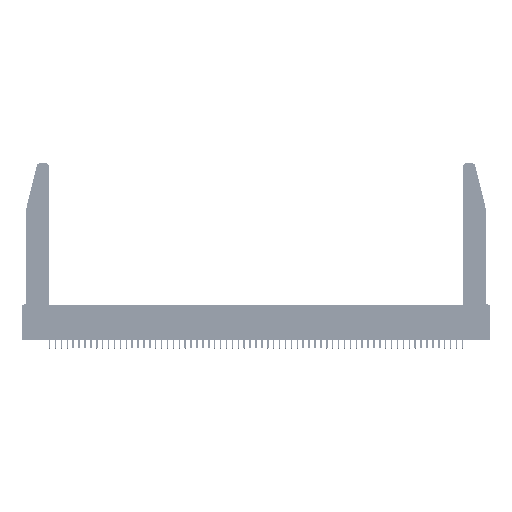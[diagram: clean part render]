
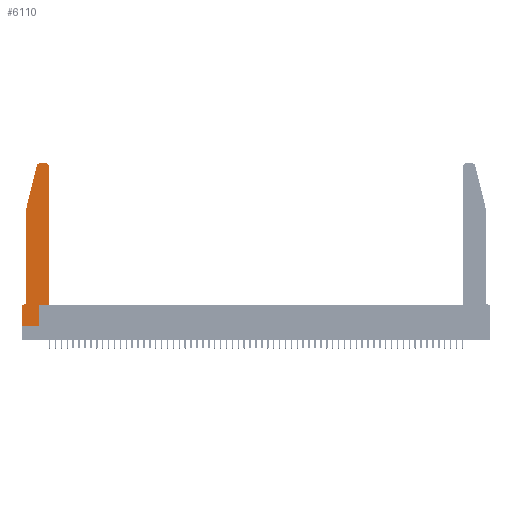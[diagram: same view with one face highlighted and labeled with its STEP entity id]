
A CAD part, top view. The second image highlights one B-rep face of the part: STEP entity #6110.
In plain terms, the highlighted planar face has unit normal (0, 0, 1).
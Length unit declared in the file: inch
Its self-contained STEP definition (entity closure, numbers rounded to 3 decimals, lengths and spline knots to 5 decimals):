
#269 = CARTESIAN_POINT ( 'NONE',  ( 0.0055, 0.42, 0.37 ) ) ;
#1552 = CARTESIAN_POINT ( 'NONE',  ( 0., 0., 0.37 ) ) ;
#1593 = DIRECTION ( 'NONE',  ( 1., 0., 0. ) ) ;
#1777 = ORIENTED_EDGE ( 'NONE', *, *, #32491, .T. ) ;
#1804 = CARTESIAN_POINT ( 'NONE',  ( 0.2865, 0.35, 0.37 ) ) ;
#2118 = VERTEX_POINT ( 'NONE', #39804 ) ;
#2926 = EDGE_CURVE ( 'NONE', #52305, #33235, #49611, .T. ) ;
#4724 = DIRECTION ( 'NONE',  ( -1., 0., 0. ) ) ;
#5284 = CARTESIAN_POINT ( 'NONE',  ( 0.4505, 2.72, 0.37 ) ) ;
#5709 = EDGE_CURVE ( 'NONE', #37300, #2118, #21955, .T. ) ;
#5731 = DIRECTION ( 'NONE',  ( -0.239, -0.971, 0. ) ) ;
#6020 = CARTESIAN_POINT ( 'NONE',  ( 0.284, 2.72, 0.37 ) ) ;
#6110 = ADVANCED_FACE ( 'NONE', ( #21896 ), #30469, .T. ) ;
#6280 = ORIENTED_EDGE ( 'NONE', *, *, #5709, .T. ) ;
#7182 = ORIENTED_EDGE ( 'NONE', *, *, #50861, .T. ) ;
#8205 = CARTESIAN_POINT ( 'NONE',  ( 0.4505, 0.35, 0.37 ) ) ;
#8643 = DIRECTION ( 'NONE',  ( 0., 0., 1. ) ) ;
#8698 = VECTOR ( 'NONE', #23076, 39.37008 ) ;
#10059 = LINE ( 'NONE', #27499, #8698 ) ;
#10401 = DIRECTION ( 'NONE',  ( 1., 0., 0. ) ) ;
#11007 = ORIENTED_EDGE ( 'NONE', *, *, #17487, .T. ) ;
#11427 = CARTESIAN_POINT ( 'NONE',  ( 0.25487, 2.72718, 0.37 ) ) ;
#12395 = LINE ( 'NONE', #8205, #22644 ) ;
#12562 = DIRECTION ( 'NONE',  ( 0., 1., 0. ) ) ;
#13392 = VECTOR ( 'NONE', #5731, 39.37008 ) ;
#13695 = CARTESIAN_POINT ( 'NONE',  ( 0.2865, 0.35, 0.37 ) ) ;
#14216 = ORIENTED_EDGE ( 'NONE', *, *, #37200, .T. ) ;
#14345 = LINE ( 'NONE', #44198, #24611 ) ;
#14688 = EDGE_LOOP ( 'NONE', ( #11007, #30832, #22617, #28702, #14216, #19615, #7182, #6280, #21599, #38607, #56515, #1777 ) ) ;
#16716 = DIRECTION ( 'NONE',  ( 1., 0., 0. ) ) ;
#17437 = VERTEX_POINT ( 'NONE', #35310 ) ;
#17487 = EDGE_CURVE ( 'NONE', #32050, #53850, #14345, .T. ) ;
#17672 = AXIS2_PLACEMENT_3D ( 'NONE', #53911, #27817, #1593 ) ;
#18965 = DIRECTION ( 'NONE',  ( 1., 0., 0. ) ) ;
#19210 = CIRCLE ( 'NONE', #37378, 0.07 ) ;
#19615 = ORIENTED_EDGE ( 'NONE', *, *, #27882, .T. ) ;
#20048 = CARTESIAN_POINT ( 'NONE',  ( 0., 0., 0.37 ) ) ;
#20575 = CARTESIAN_POINT ( 'NONE',  ( 0.0755, 0.35, 0.37 ) ) ;
#21590 = AXIS2_PLACEMENT_3D ( 'NONE', #6020, #36625, #10401 ) ;
#21599 = ORIENTED_EDGE ( 'NONE', *, *, #23009, .T. ) ;
#21896 = FACE_OUTER_BOUND ( 'NONE', #14688, .T. ) ;
#21955 = LINE ( 'NONE', #1552, #32270 ) ;
#22404 = DIRECTION ( 'NONE',  ( -1., 0., 0. ) ) ;
#22617 = ORIENTED_EDGE ( 'NONE', *, *, #2926, .T. ) ;
#22644 = VECTOR ( 'NONE', #12562, 39.37008 ) ;
#23009 = EDGE_CURVE ( 'NONE', #2118, #51243, #48115, .T. ) ;
#23076 = DIRECTION ( 'NONE',  ( 0., -1., 0. ) ) ;
#23194 = VECTOR ( 'NONE', #24442, 39.37008 ) ;
#24442 = DIRECTION ( 'NONE',  ( 0., -1., 0. ) ) ;
#24611 = VECTOR ( 'NONE', #22404, 39.37008 ) ;
#24880 = CIRCLE ( 'NONE', #17672, 0.03 ) ;
#25055 = LINE ( 'NONE', #38556, #35394 ) ;
#26169 = CIRCLE ( 'NONE', #21590, 0.03 ) ;
#27122 = CARTESIAN_POINT ( 'NONE',  ( 0.4505, 0.35, 0.37 ) ) ;
#27401 = LINE ( 'NONE', #20575, #39040 ) ;
#27499 = CARTESIAN_POINT ( 'NONE',  ( 0.0755, 2., 0.37 ) ) ;
#27817 = DIRECTION ( 'NONE',  ( 0., 0., 1. ) ) ;
#27882 = EDGE_CURVE ( 'NONE', #50797, #43122, #27401, .T. ) ;
#28244 = VERTEX_POINT ( 'NONE', #5284 ) ;
#28702 = ORIENTED_EDGE ( 'NONE', *, *, #33730, .T. ) ;
#30469 = PLANE ( 'NONE',  #50492 ) ;
#30832 = ORIENTED_EDGE ( 'NONE', *, *, #48964, .T. ) ;
#30971 = DIRECTION ( 'NONE',  ( 0., 0., -1. ) ) ;
#31197 = CARTESIAN_POINT ( 'NONE',  ( 0.284, 2.75, 0.37 ) ) ;
#32050 = VERTEX_POINT ( 'NONE', #38021 ) ;
#32270 = VECTOR ( 'NONE', #18965, 39.37008 ) ;
#32491 = EDGE_CURVE ( 'NONE', #28244, #32050, #24880, .T. ) ;
#33235 = VERTEX_POINT ( 'NONE', #41688 ) ;
#33644 = VERTEX_POINT ( 'NONE', #27122 ) ;
#33730 = EDGE_CURVE ( 'NONE', #33235, #17437, #10059, .T. ) ;
#34872 = CARTESIAN_POINT ( 'NONE',  ( 0., 0.35, 0.37 ) ) ;
#35310 = CARTESIAN_POINT ( 'NONE',  ( 0.0755, 0.42, 0.37 ) ) ;
#35394 = VECTOR ( 'NONE', #16716, 39.37008 ) ;
#36329 = CARTESIAN_POINT ( 'NONE',  ( 0.0755, 2., 0.37 ) ) ;
#36553 = VECTOR ( 'NONE', #41215, 39.37008 ) ;
#36625 = DIRECTION ( 'NONE',  ( 0., 0., 1. ) ) ;
#37200 = EDGE_CURVE ( 'NONE', #17437, #50797, #19210, .T. ) ;
#37300 = VERTEX_POINT ( 'NONE', #40097 ) ;
#37378 = AXIS2_PLACEMENT_3D ( 'NONE', #269, #30971, #4724 ) ;
#38021 = CARTESIAN_POINT ( 'NONE',  ( 0.4205, 2.75, 0.37 ) ) ;
#38172 = CARTESIAN_POINT ( 'NONE',  ( 0., 0.35, 0.37 ) ) ;
#38556 = CARTESIAN_POINT ( 'NONE',  ( 0.4505, 0.35, 0.37 ) ) ;
#38607 = ORIENTED_EDGE ( 'NONE', *, *, #46772, .T. ) ;
#39040 = VECTOR ( 'NONE', #51116, 39.37008 ) ;
#39230 = DIRECTION ( 'NONE',  ( 1., 0., 0. ) ) ;
#39804 = CARTESIAN_POINT ( 'NONE',  ( 0.2865, 0., 0.37 ) ) ;
#40097 = CARTESIAN_POINT ( 'NONE',  ( 0., 0., 0.37 ) ) ;
#41215 = DIRECTION ( 'NONE',  ( 0., 1., 0. ) ) ;
#41688 = CARTESIAN_POINT ( 'NONE',  ( 0.0755, 2., 0.37 ) ) ;
#43122 = VERTEX_POINT ( 'NONE', #38172 ) ;
#44198 = CARTESIAN_POINT ( 'NONE',  ( 0.2605, 2.75, 0.37 ) ) ;
#45011 = EDGE_CURVE ( 'NONE', #33644, #28244, #12395, .T. ) ;
#45603 = LINE ( 'NONE', #20048, #23194 ) ;
#46772 = EDGE_CURVE ( 'NONE', #51243, #33644, #25055, .T. ) ;
#48115 = LINE ( 'NONE', #1804, #36553 ) ;
#48964 = EDGE_CURVE ( 'NONE', #53850, #52305, #26169, .T. ) ;
#49436 = CARTESIAN_POINT ( 'NONE',  ( 0.0055, 0.35, 0.37 ) ) ;
#49611 = LINE ( 'NONE', #36329, #13392 ) ;
#50492 = AXIS2_PLACEMENT_3D ( 'NONE', #34872, #8643, #39230 ) ;
#50797 = VERTEX_POINT ( 'NONE', #49436 ) ;
#50861 = EDGE_CURVE ( 'NONE', #43122, #37300, #45603, .T. ) ;
#51116 = DIRECTION ( 'NONE',  ( -1., 0., 0. ) ) ;
#51243 = VERTEX_POINT ( 'NONE', #13695 ) ;
#52305 = VERTEX_POINT ( 'NONE', #11427 ) ;
#53850 = VERTEX_POINT ( 'NONE', #31197 ) ;
#53911 = CARTESIAN_POINT ( 'NONE',  ( 0.4205, 2.72, 0.37 ) ) ;
#56515 = ORIENTED_EDGE ( 'NONE', *, *, #45011, .T. ) ;
